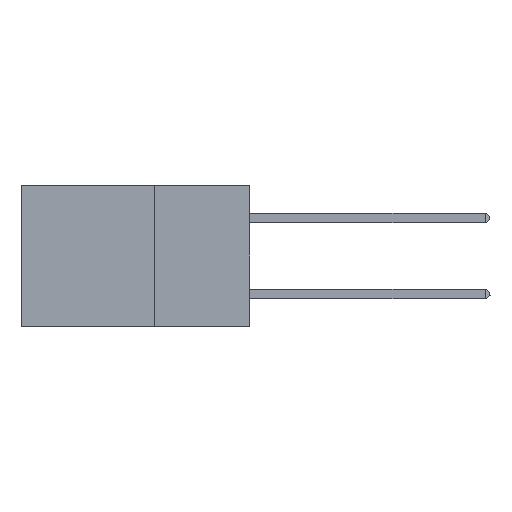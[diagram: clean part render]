
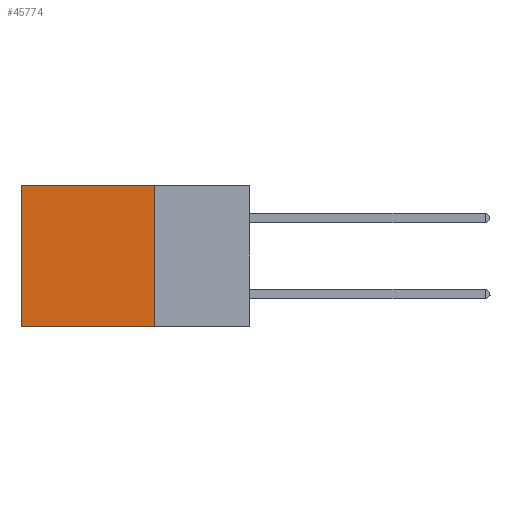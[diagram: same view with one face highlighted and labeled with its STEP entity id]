
A CAD part, left-side view. The second image highlights one B-rep face of the part: STEP entity #45774.
In plain terms, the highlighted planar face has unit normal (-1, 0, 0).
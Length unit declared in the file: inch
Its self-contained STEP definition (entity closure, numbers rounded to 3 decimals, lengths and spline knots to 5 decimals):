
#89 = EDGE_CURVE ( 'NONE', #14617, #44028, #41167, .T. ) ;
#1270 = DIRECTION ( 'NONE',  ( 0., 1., 0. ) ) ;
#3299 = CARTESIAN_POINT ( 'NONE',  ( 0.2875, 0.6, 0. ) ) ;
#3797 = CARTESIAN_POINT ( 'NONE',  ( 0.2875, 0.25, 0. ) ) ;
#5711 = CARTESIAN_POINT ( 'NONE',  ( 0.2875, 0.6, -0.37 ) ) ;
#7718 = DIRECTION ( 'NONE',  ( 0., 0., -1. ) ) ;
#8012 = LINE ( 'NONE', #3299, #26313 ) ;
#8892 = DIRECTION ( 'NONE',  ( 1., 0., 0. ) ) ;
#9425 = ORIENTED_EDGE ( 'NONE', *, *, #33973, .F. ) ;
#9566 = EDGE_CURVE ( 'NONE', #34687, #44028, #8012, .T. ) ;
#12505 = DIRECTION ( 'NONE',  ( 0., 1., 0. ) ) ;
#12870 = VECTOR ( 'NONE', #1270, 39.37008 ) ;
#13618 = LINE ( 'NONE', #30564, #30590 ) ;
#14347 = CARTESIAN_POINT ( 'NONE',  ( 0.2875, 0.25, 0. ) ) ;
#14617 = VERTEX_POINT ( 'NONE', #37762 ) ;
#19752 = PLANE ( 'NONE',  #42978 ) ;
#22616 = EDGE_LOOP ( 'NONE', ( #29206, #37152, #9425, #34611 ) ) ;
#25665 = LINE ( 'NONE', #3797, #42996 ) ;
#26313 = VECTOR ( 'NONE', #46230, 39.37008 ) ;
#26831 = CARTESIAN_POINT ( 'NONE',  ( 0.2875, 0.6, 0. ) ) ;
#27192 = CARTESIAN_POINT ( 'NONE',  ( 0.2875, 0.25, -0.37 ) ) ;
#29206 = ORIENTED_EDGE ( 'NONE', *, *, #9566, .T. ) ;
#30564 = CARTESIAN_POINT ( 'NONE',  ( 0.2875, 0.25, 0. ) ) ;
#30590 = VECTOR ( 'NONE', #12505, 39.37008 ) ;
#32307 = EDGE_CURVE ( 'NONE', #38198, #34687, #13618, .T. ) ;
#33973 = EDGE_CURVE ( 'NONE', #38198, #14617, #25665, .T. ) ;
#34088 = DIRECTION ( 'NONE',  ( 0., 0., -1. ) ) ;
#34611 = ORIENTED_EDGE ( 'NONE', *, *, #32307, .T. ) ;
#34687 = VERTEX_POINT ( 'NONE', #26831 ) ;
#37152 = ORIENTED_EDGE ( 'NONE', *, *, #89, .F. ) ;
#37762 = CARTESIAN_POINT ( 'NONE',  ( 0.2875, 0.25, -0.37 ) ) ;
#37983 = FACE_OUTER_BOUND ( 'NONE', #22616, .T. ) ;
#38198 = VERTEX_POINT ( 'NONE', #14347 ) ;
#40824 = CARTESIAN_POINT ( 'NONE',  ( 0.2875, 0.25, 0. ) ) ;
#41167 = LINE ( 'NONE', #27192, #12870 ) ;
#42978 = AXIS2_PLACEMENT_3D ( 'NONE', #40824, #8892, #34088 ) ;
#42996 = VECTOR ( 'NONE', #7718, 39.37008 ) ;
#44028 = VERTEX_POINT ( 'NONE', #5711 ) ;
#45774 = ADVANCED_FACE ( 'NONE', ( #37983 ), #19752, .F. ) ;
#46230 = DIRECTION ( 'NONE',  ( 0., 0., -1. ) ) ;
